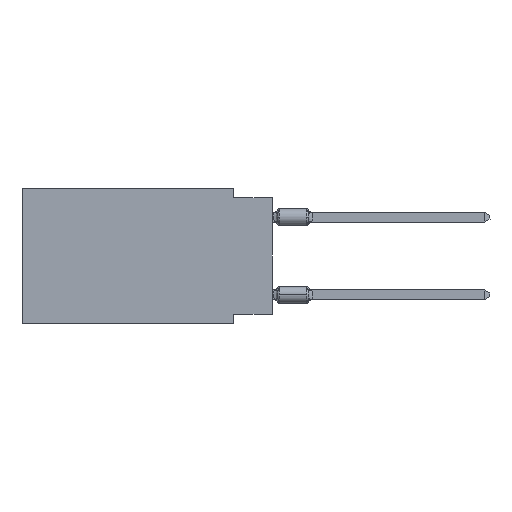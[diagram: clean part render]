
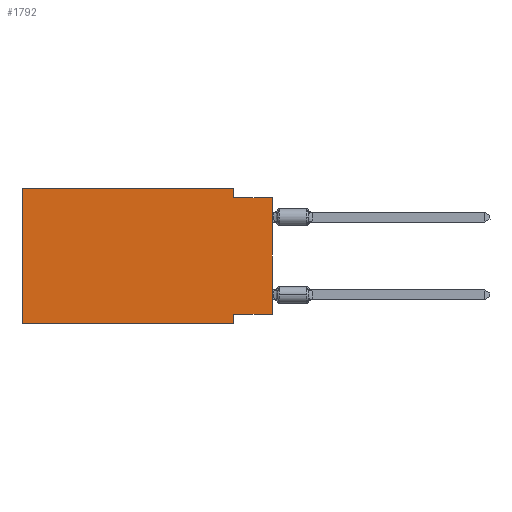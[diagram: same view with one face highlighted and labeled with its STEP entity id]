
A CAD part, left-side view. The second image highlights one B-rep face of the part: STEP entity #1792.
In plain terms, the highlighted planar face has unit normal (-1, 0, 0).
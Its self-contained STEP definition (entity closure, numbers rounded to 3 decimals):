
#72 = FACE_OUTER_BOUND ( 'NONE', #9429, .T. ) ;
#175 = CARTESIAN_POINT ( 'NONE',  ( 0., 0., -8.255 ) ) ;
#409 = VECTOR ( 'NONE', #2957, 1000. ) ;
#1120 = CARTESIAN_POINT ( 'NONE',  ( 0., 16.383, -8.89 ) ) ;
#1309 = VERTEX_POINT ( 'NONE', #11764 ) ;
#1644 = VECTOR ( 'NONE', #9152, 1000. ) ;
#1792 = ADVANCED_FACE ( 'NONE', ( #72 ), #5208, .F. ) ;
#1877 = LINE ( 'NONE', #15774, #10123 ) ;
#2085 = EDGE_CURVE ( 'NONE', #1309, #4125, #13310, .T. ) ;
#2280 = DIRECTION ( 'NONE',  ( 0., -1., 0. ) ) ;
#2889 = CARTESIAN_POINT ( 'NONE',  ( 0., 0., -8.255 ) ) ;
#2957 = DIRECTION ( 'NONE',  ( 0., 0., -1. ) ) ;
#3304 = LINE ( 'NONE', #16367, #3605 ) ;
#3512 = ORIENTED_EDGE ( 'NONE', *, *, #7388, .T. ) ;
#3605 = VECTOR ( 'NONE', #13498, 1000. ) ;
#3713 = CARTESIAN_POINT ( 'NONE',  ( 0., 16.383, 0. ) ) ;
#4125 = VERTEX_POINT ( 'NONE', #13269 ) ;
#4193 = VERTEX_POINT ( 'NONE', #12270 ) ;
#4221 = DIRECTION ( 'NONE',  ( 0., 1., 0. ) ) ;
#4321 = ORIENTED_EDGE ( 'NONE', *, *, #10549, .F. ) ;
#4999 = DIRECTION ( 'NONE',  ( 0., -1., 0. ) ) ;
#5073 = VERTEX_POINT ( 'NONE', #6269 ) ;
#5208 = PLANE ( 'NONE',  #15662 ) ;
#5599 = ORIENTED_EDGE ( 'NONE', *, *, #11124, .T. ) ;
#5808 = VECTOR ( 'NONE', #4999, 1000. ) ;
#6242 = CARTESIAN_POINT ( 'NONE',  ( 0., 16.383, 0. ) ) ;
#6269 = CARTESIAN_POINT ( 'NONE',  ( 0., 2.54, -8.89 ) ) ;
#6672 = VERTEX_POINT ( 'NONE', #1120 ) ;
#6781 = LINE ( 'NONE', #14549, #12115 ) ;
#7077 = EDGE_CURVE ( 'NONE', #4125, #7809, #16513, .T. ) ;
#7388 = EDGE_CURVE ( 'NONE', #6672, #5073, #6781, .T. ) ;
#7809 = VERTEX_POINT ( 'NONE', #12429 ) ;
#8242 = CARTESIAN_POINT ( 'NONE',  ( 0., 16.383, 0. ) ) ;
#8266 = EDGE_CURVE ( 'NONE', #4193, #5073, #3304, .T. ) ;
#9152 = DIRECTION ( 'NONE',  ( 0., 0., 1. ) ) ;
#9429 = EDGE_LOOP ( 'NONE', ( #5599, #15032, #16002, #4321, #13478, #3512, #10093, #14702 ) ) ;
#9525 = DIRECTION ( 'NONE',  ( 0., -1., 0. ) ) ;
#10093 = ORIENTED_EDGE ( 'NONE', *, *, #8266, .F. ) ;
#10123 = VECTOR ( 'NONE', #12139, 1000. ) ;
#10303 = DIRECTION ( 'NONE',  ( 1., 0., 0. ) ) ;
#10518 = CARTESIAN_POINT ( 'NONE',  ( 0., 16.383, 0. ) ) ;
#10549 = EDGE_CURVE ( 'NONE', #13117, #1309, #15033, .T. ) ;
#10652 = LINE ( 'NONE', #2889, #13831 ) ;
#11124 = EDGE_CURVE ( 'NONE', #12173, #7809, #1877, .T. ) ;
#11764 = CARTESIAN_POINT ( 'NONE',  ( 0., 2.54, 0. ) ) ;
#11971 = CARTESIAN_POINT ( 'NONE',  ( 0., 2.54, 0. ) ) ;
#12115 = VECTOR ( 'NONE', #9525, 1000. ) ;
#12139 = DIRECTION ( 'NONE',  ( 0., 0., 1. ) ) ;
#12173 = VERTEX_POINT ( 'NONE', #175 ) ;
#12270 = CARTESIAN_POINT ( 'NONE',  ( 0., 2.54, -8.255 ) ) ;
#12429 = CARTESIAN_POINT ( 'NONE',  ( 0., 0., -0.635 ) ) ;
#13117 = VERTEX_POINT ( 'NONE', #10518 ) ;
#13269 = CARTESIAN_POINT ( 'NONE',  ( 0., 2.54, -0.635 ) ) ;
#13310 = LINE ( 'NONE', #11971, #409 ) ;
#13326 = LINE ( 'NONE', #8242, #1644 ) ;
#13373 = EDGE_CURVE ( 'NONE', #6672, #13117, #13326, .T. ) ;
#13478 = ORIENTED_EDGE ( 'NONE', *, *, #13373, .F. ) ;
#13498 = DIRECTION ( 'NONE',  ( 0., 0., -1. ) ) ;
#13831 = VECTOR ( 'NONE', #4221, 1000. ) ;
#14251 = VECTOR ( 'NONE', #2280, 1000. ) ;
#14549 = CARTESIAN_POINT ( 'NONE',  ( 0., 16.383, -8.89 ) ) ;
#14582 = EDGE_CURVE ( 'NONE', #12173, #4193, #10652, .T. ) ;
#14702 = ORIENTED_EDGE ( 'NONE', *, *, #14582, .F. ) ;
#15032 = ORIENTED_EDGE ( 'NONE', *, *, #7077, .F. ) ;
#15033 = LINE ( 'NONE', #6242, #5808 ) ;
#15252 = CARTESIAN_POINT ( 'NONE',  ( 0., 0., -0.635 ) ) ;
#15418 = DIRECTION ( 'NONE',  ( 0., 0., -1. ) ) ;
#15662 = AXIS2_PLACEMENT_3D ( 'NONE', #3713, #10303, #15418 ) ;
#15774 = CARTESIAN_POINT ( 'NONE',  ( 0., 0., 0. ) ) ;
#16002 = ORIENTED_EDGE ( 'NONE', *, *, #2085, .F. ) ;
#16367 = CARTESIAN_POINT ( 'NONE',  ( 0., 2.54, -8.89 ) ) ;
#16513 = LINE ( 'NONE', #15252, #14251 ) ;
